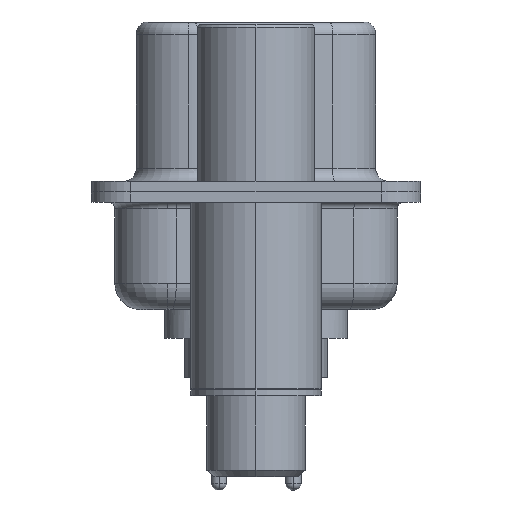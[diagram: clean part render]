
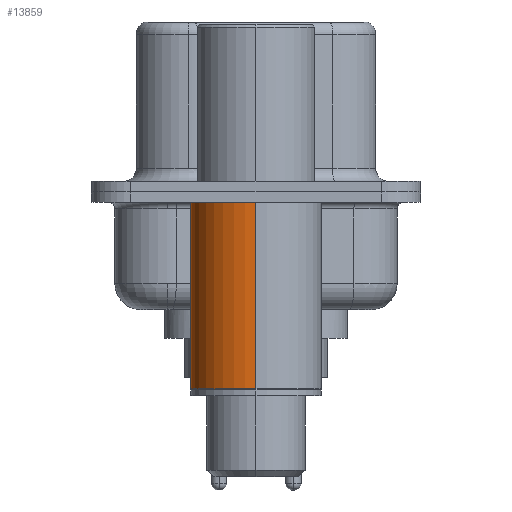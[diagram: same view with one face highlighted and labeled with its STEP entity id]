
A CAD part, left-side view. The second image highlights one B-rep face of the part: STEP entity #13859.
In plain terms, the highlighted cylindrical face has radius 2.5 mm (diameter 5 mm), a partial arc.
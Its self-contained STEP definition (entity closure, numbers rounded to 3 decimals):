
#55 = VECTOR ( 'NONE', #24621, 1000. ) ;
#616 = DIRECTION ( 'NONE',  ( 0., 0., 1. ) ) ;
#1354 = CIRCLE ( 'NONE', #23300, 2.5 ) ;
#1449 = EDGE_CURVE ( 'NONE', #5780, #14881, #23476, .T. ) ;
#2425 = CARTESIAN_POINT ( 'NONE',  ( 2.5, 0., -7.525 ) ) ;
#3416 = EDGE_CURVE ( 'NONE', #8314, #6558, #1354, .T. ) ;
#3763 = DIRECTION ( 'NONE',  ( 1., 0., 0. ) ) ;
#3810 = DIRECTION ( 'NONE',  ( 0., 0., 1. ) ) ;
#3891 = CARTESIAN_POINT ( 'NONE',  ( 0., 0., -0.4 ) ) ;
#4326 = ORIENTED_EDGE ( 'NONE', *, *, #3416, .F. ) ;
#5479 = AXIS2_PLACEMENT_3D ( 'NONE', #15003, #22897, #24876 ) ;
#5780 = VERTEX_POINT ( 'NONE', #2425 ) ;
#5921 = LINE ( 'NONE', #8982, #55 ) ;
#6558 = VERTEX_POINT ( 'NONE', #9278 ) ;
#7300 = LINE ( 'NONE', #12370, #16454 ) ;
#7573 = ORIENTED_EDGE ( 'NONE', *, *, #1449, .T. ) ;
#8314 = VERTEX_POINT ( 'NONE', #23333 ) ;
#8362 = AXIS2_PLACEMENT_3D ( 'NONE', #19698, #19526, #19356 ) ;
#8982 = CARTESIAN_POINT ( 'NONE',  ( 2.5, 0., 0.581 ) ) ;
#9278 = CARTESIAN_POINT ( 'NONE',  ( -2.5, 0., -0.4 ) ) ;
#10321 = ORIENTED_EDGE ( 'NONE', *, *, #24746, .T. ) ;
#12370 = CARTESIAN_POINT ( 'NONE',  ( -2.5, 0., 0.581 ) ) ;
#13859 = ADVANCED_FACE ( 'NONE', ( #18173 ), #21543, .T. ) ;
#14881 = VERTEX_POINT ( 'NONE', #18489 ) ;
#15003 = CARTESIAN_POINT ( 'NONE',  ( 0., 0., 0.581 ) ) ;
#16454 = VECTOR ( 'NONE', #616, 1000. ) ;
#18173 = FACE_OUTER_BOUND ( 'NONE', #22537, .T. ) ;
#18489 = CARTESIAN_POINT ( 'NONE',  ( -2.5, 0., -7.525 ) ) ;
#19217 = ORIENTED_EDGE ( 'NONE', *, *, #20583, .F. ) ;
#19356 = DIRECTION ( 'NONE',  ( 1., 0., 0. ) ) ;
#19526 = DIRECTION ( 'NONE',  ( 0., 0., 1. ) ) ;
#19698 = CARTESIAN_POINT ( 'NONE',  ( 0., 0., -7.525 ) ) ;
#20583 = EDGE_CURVE ( 'NONE', #5780, #8314, #5921, .T. ) ;
#21543 = CYLINDRICAL_SURFACE ( 'NONE', #5479, 2.5 ) ;
#22537 = EDGE_LOOP ( 'NONE', ( #7573, #10321, #4326, #19217 ) ) ;
#22897 = DIRECTION ( 'NONE',  ( 0., 0., 1. ) ) ;
#23300 = AXIS2_PLACEMENT_3D ( 'NONE', #3891, #3810, #3763 ) ;
#23333 = CARTESIAN_POINT ( 'NONE',  ( 2.5, 0., -0.4 ) ) ;
#23476 = CIRCLE ( 'NONE', #8362, 2.5 ) ;
#24621 = DIRECTION ( 'NONE',  ( 0., 0., 1. ) ) ;
#24746 = EDGE_CURVE ( 'NONE', #14881, #6558, #7300, .T. ) ;
#24876 = DIRECTION ( 'NONE',  ( 1., 0., 0. ) ) ;
